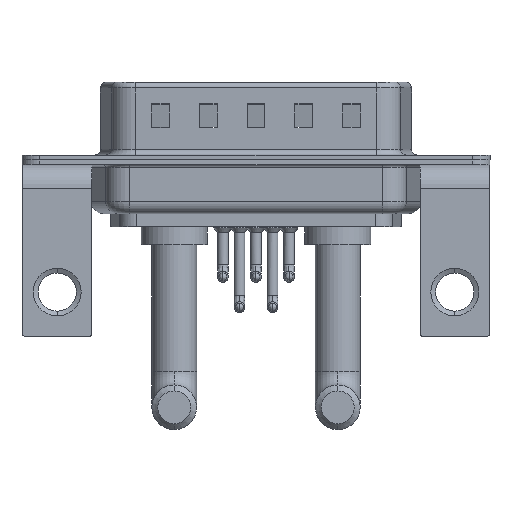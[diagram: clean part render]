
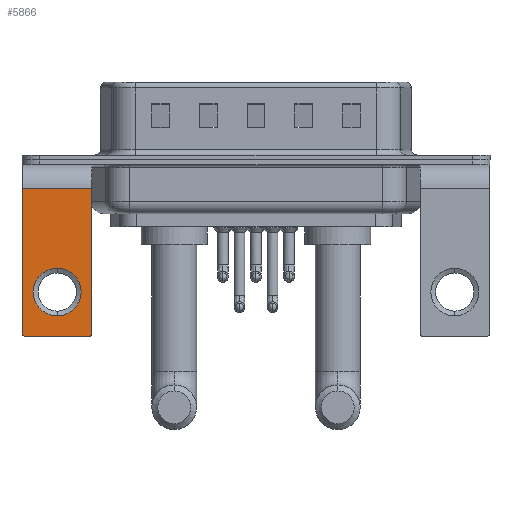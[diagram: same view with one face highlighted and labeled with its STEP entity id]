
A CAD part, front view. The second image highlights one B-rep face of the part: STEP entity #5866.
In plain terms, the highlighted planar face has unit normal (0, -1, 0).
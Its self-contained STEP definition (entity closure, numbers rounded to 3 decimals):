
#382 = VERTEX_POINT ( 'NONE', #696 ) ;
#384 = VECTOR ( 'NONE', #16405, 1000. ) ;
#628 = DIRECTION ( 'NONE',  ( 0., 0., 1. ) ) ;
#696 = CARTESIAN_POINT ( 'NONE',  ( -2.65, -6.25, -14.8 ) ) ;
#1078 = CIRCLE ( 'NONE', #10900, 2. ) ;
#1228 = EDGE_CURVE ( 'NONE', #17860, #14567, #5917, .T. ) ;
#1356 = DIRECTION ( 'NONE',  ( 0., 0., 1. ) ) ;
#1414 = EDGE_CURVE ( 'NONE', #8487, #5396, #4876, .T. ) ;
#1456 = CARTESIAN_POINT ( 'NONE',  ( 0., -6.25, -11.07 ) ) ;
#1532 = FACE_OUTER_BOUND ( 'NONE', #16967, .T. ) ;
#1571 = DIRECTION ( 'NONE',  ( 0., 1., 0. ) ) ;
#1946 = CARTESIAN_POINT ( 'NONE',  ( -2.65, -6.25, -14.55 ) ) ;
#1969 = ORIENTED_EDGE ( 'NONE', *, *, #8495, .F. ) ;
#2178 = VERTEX_POINT ( 'NONE', #9346 ) ;
#2271 = CARTESIAN_POINT ( 'NONE',  ( 2.65, -6.25, -14.55 ) ) ;
#4751 = DIRECTION ( 'NONE',  ( 0., 0., -1. ) ) ;
#4826 = DIRECTION ( 'NONE',  ( 0., 0., 1. ) ) ;
#4876 = LINE ( 'NONE', #16505, #384 ) ;
#4960 = CARTESIAN_POINT ( 'NONE',  ( -2.9, -6.25, -2.4 ) ) ;
#5396 = VERTEX_POINT ( 'NONE', #4960 ) ;
#5866 = ADVANCED_FACE ( 'NONE', ( #16561, #1532 ), #19873, .F. ) ;
#5917 = CIRCLE ( 'NONE', #6605, 0.25 ) ;
#6329 = ORIENTED_EDGE ( 'NONE', *, *, #9209, .T. ) ;
#6505 = CARTESIAN_POINT ( 'NONE',  ( 2.9, -6.25, -2.4 ) ) ;
#6605 = AXIS2_PLACEMENT_3D ( 'NONE', #2271, #17087, #12053 ) ;
#7766 = EDGE_CURVE ( 'NONE', #13915, #382, #18612, .T. ) ;
#7830 = AXIS2_PLACEMENT_3D ( 'NONE', #12013, #17051, #8703 ) ;
#8487 = VERTEX_POINT ( 'NONE', #6505 ) ;
#8495 = EDGE_CURVE ( 'NONE', #8487, #14567, #18347, .T. ) ;
#8703 = DIRECTION ( 'NONE',  ( 0., 0., 1. ) ) ;
#8752 = ORIENTED_EDGE ( 'NONE', *, *, #1414, .T. ) ;
#9209 = EDGE_CURVE ( 'NONE', #19562, #2178, #1078, .T. ) ;
#9346 = CARTESIAN_POINT ( 'NONE',  ( 0., -6.25, -13.07 ) ) ;
#10078 = VECTOR ( 'NONE', #14566, 1000. ) ;
#10442 = CARTESIAN_POINT ( 'NONE',  ( -2.9, -6.25, -2.4 ) ) ;
#10556 = AXIS2_PLACEMENT_3D ( 'NONE', #14817, #13070, #4826 ) ;
#10620 = DIRECTION ( 'NONE',  ( 0., -1., 0. ) ) ;
#10839 = LINE ( 'NONE', #10442, #19368 ) ;
#10842 = CARTESIAN_POINT ( 'NONE',  ( 2.9, -6.25, -14.55 ) ) ;
#10900 = AXIS2_PLACEMENT_3D ( 'NONE', #1456, #1571, #1356 ) ;
#11138 = ORIENTED_EDGE ( 'NONE', *, *, #19918, .F. ) ;
#11388 = CARTESIAN_POINT ( 'NONE',  ( 2.9, -6.25, -14.8 ) ) ;
#12013 = CARTESIAN_POINT ( 'NONE',  ( 0., -6.25, -11.07 ) ) ;
#12049 = CIRCLE ( 'NONE', #7830, 2. ) ;
#12053 = DIRECTION ( 'NONE',  ( 0., 0., 1. ) ) ;
#13070 = DIRECTION ( 'NONE',  ( 0., 1., 0. ) ) ;
#13622 = EDGE_CURVE ( 'NONE', #2178, #19562, #12049, .T. ) ;
#13627 = ORIENTED_EDGE ( 'NONE', *, *, #21168, .T. ) ;
#13711 = AXIS2_PLACEMENT_3D ( 'NONE', #1946, #10620, #628 ) ;
#13915 = VERTEX_POINT ( 'NONE', #21519 ) ;
#14566 = DIRECTION ( 'NONE',  ( -1., 0., 0. ) ) ;
#14567 = VERTEX_POINT ( 'NONE', #10842 ) ;
#14817 = CARTESIAN_POINT ( 'NONE',  ( 2.9, -6.25, -2.4 ) ) ;
#14828 = ORIENTED_EDGE ( 'NONE', *, *, #13622, .T. ) ;
#15283 = ORIENTED_EDGE ( 'NONE', *, *, #7766, .T. ) ;
#16024 = CARTESIAN_POINT ( 'NONE',  ( 2.65, -6.25, -14.8 ) ) ;
#16405 = DIRECTION ( 'NONE',  ( -1., 0., 0. ) ) ;
#16505 = CARTESIAN_POINT ( 'NONE',  ( 2.9, -6.25, -2.4 ) ) ;
#16561 = FACE_BOUND ( 'NONE', #20298, .T. ) ;
#16967 = EDGE_LOOP ( 'NONE', ( #13627, #15283, #11138, #17403, #1969, #8752 ) ) ;
#17051 = DIRECTION ( 'NONE',  ( 0., 1., 0. ) ) ;
#17087 = DIRECTION ( 'NONE',  ( 0., -1., 0. ) ) ;
#17403 = ORIENTED_EDGE ( 'NONE', *, *, #1228, .T. ) ;
#17763 = CARTESIAN_POINT ( 'NONE',  ( 0., -6.25, -9.07 ) ) ;
#17839 = LINE ( 'NONE', #11388, #10078 ) ;
#17860 = VERTEX_POINT ( 'NONE', #16024 ) ;
#18347 = LINE ( 'NONE', #19791, #20405 ) ;
#18612 = CIRCLE ( 'NONE', #13711, 0.25 ) ;
#19187 = DIRECTION ( 'NONE',  ( 0., 0., -1. ) ) ;
#19368 = VECTOR ( 'NONE', #19187, 1000. ) ;
#19562 = VERTEX_POINT ( 'NONE', #17763 ) ;
#19791 = CARTESIAN_POINT ( 'NONE',  ( 2.9, -6.25, -2.4 ) ) ;
#19873 = PLANE ( 'NONE',  #10556 ) ;
#19918 = EDGE_CURVE ( 'NONE', #17860, #382, #17839, .T. ) ;
#20298 = EDGE_LOOP ( 'NONE', ( #14828, #6329 ) ) ;
#20405 = VECTOR ( 'NONE', #4751, 1000. ) ;
#21168 = EDGE_CURVE ( 'NONE', #5396, #13915, #10839, .T. ) ;
#21519 = CARTESIAN_POINT ( 'NONE',  ( -2.9, -6.25, -14.55 ) ) ;
